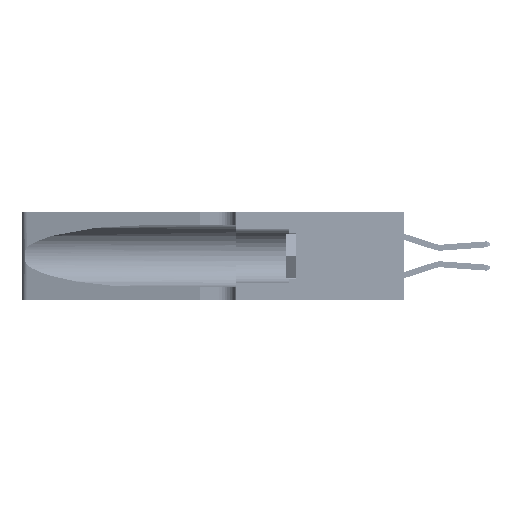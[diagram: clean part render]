
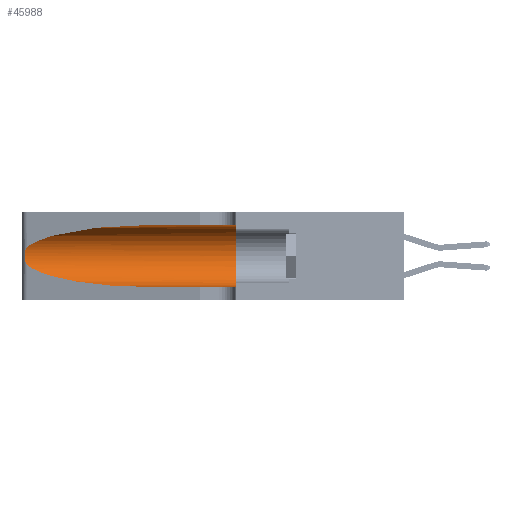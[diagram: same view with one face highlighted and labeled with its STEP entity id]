
A CAD part, left-side view. The second image highlights one B-rep face of the part: STEP entity #45988.
In plain terms, the highlighted cylindrical face has radius 3.308 mm (diameter 6.617 mm), a partial arc.
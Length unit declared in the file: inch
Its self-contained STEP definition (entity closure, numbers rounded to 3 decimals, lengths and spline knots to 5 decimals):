
#150 = CARTESIAN_POINT ( 'NONE',  ( 0.1305, 0.72297, 0.05475 ) ) ;
#905 = CARTESIAN_POINT ( 'NONE',  ( 0.25487, 1.22718, 0.14631 ) ) ;
#2768 = DIRECTION ( 'NONE',  ( 0., 0., 1. ) ) ;
#3040 = DIRECTION ( 'NONE',  ( 0., -1., 0. ) ) ;
#4184 = ORIENTED_EDGE ( 'NONE', *, *, #7627, .T. ) ;
#4466 = FACE_OUTER_BOUND ( 'NONE', #8411, .T. ) ;
#5339 = EDGE_CURVE ( 'NONE', #33217, #45054, #44253, .T. ) ;
#6113 = CARTESIAN_POINT ( 'NONE',  ( 0.25555, 1.22993, 0.14849 ) ) ;
#6825 = DIRECTION ( 'NONE',  ( 0., 0., -1. ) ) ;
#7461 = ORIENTED_EDGE ( 'NONE', *, *, #21922, .F. ) ;
#7483 = EDGE_CURVE ( 'NONE', #41468, #37640, #28538, .T. ) ;
#7627 = EDGE_CURVE ( 'NONE', #37640, #44772, #17730, .T. ) ;
#8411 = EDGE_LOOP ( 'NONE', ( #37162, #33918, #4184, #10391, #7461, #30241 ) ) ;
#8842 = DIRECTION ( 'NONE',  ( 0., -1., 0. ) ) ;
#9615 = VERTEX_POINT ( 'NONE', #32115 ) ;
#10391 = ORIENTED_EDGE ( 'NONE', *, *, #46859, .T. ) ;
#10669 = CARTESIAN_POINT ( 'NONE',  ( 0.25639, 1.23186, 0.15144 ) ) ;
#10843 = VECTOR ( 'NONE', #31134, 39.37008 ) ;
#11006 = CARTESIAN_POINT ( 'NONE',  ( 0.25555, 1.22994, 0.2215 ) ) ;
#11738 = CARTESIAN_POINT ( 'NONE',  ( 0.1305, 0.72297, 0.31525 ) ) ;
#15997 = CARTESIAN_POINT ( 'NONE',  ( 0.18966, 0.96281, 0.31525 ) ) ;
#16073 = EDGE_CURVE ( 'NONE', #33217, #41468, #32940, .T. ) ;
#16273 = VECTOR ( 'NONE', #8842, 39.37008 ) ;
#16305 = CARTESIAN_POINT ( 'NONE',  ( 0.1305, 1.61858, 0.05475 ) ) ;
#17011 = CARTESIAN_POINT ( 'NONE',  ( 0.1305, 0.72297, 0.31525 ) ) ;
#17193 = CARTESIAN_POINT ( 'NONE',  ( 0.25487, 1.22718, 0.22369 ) ) ;
#17338 = CIRCLE ( 'NONE', #37780, 0.13025 ) ;
#17730 =( BOUNDED_CURVE ( )  B_SPLINE_CURVE ( 3, ( #905, #27064, #31245, #42134 ),
 .UNSPECIFIED., .F., .F. ) 
 B_SPLINE_CURVE_WITH_KNOTS ( ( 4, 4 ),
 ( 3.44316, 4.71239 ),
 .UNSPECIFIED. ) 
 CURVE ( )  GEOMETRIC_REPRESENTATION_ITEM ( )  RATIONAL_B_SPLINE_CURVE ( ( 1., 0.87, 0.87, 1. ) ) 
 REPRESENTATION_ITEM ( '' )  );
#17924 = CARTESIAN_POINT ( 'NONE',  ( 0.1305, 1.61858, 0.185 ) ) ;
#18220 = CARTESIAN_POINT ( 'NONE',  ( 0.25789, 1.23486, 0.15765 ) ) ;
#18898 = CARTESIAN_POINT ( 'NONE',  ( 0.26017, 1.23833, 0.17102 ) ) ;
#21922 = EDGE_CURVE ( 'NONE', #45054, #9615, #17338, .T. ) ;
#22073 = CARTESIAN_POINT ( 'NONE',  ( 0.25487, 1.22718, 0.22369 ) ) ;
#22604 = CYLINDRICAL_SURFACE ( 'NONE', #29586, 0.13025 ) ;
#23156 = CARTESIAN_POINT ( 'NONE',  ( 0.25487, 1.22718, 0.22369 ) ) ;
#24676 = CARTESIAN_POINT ( 'NONE',  ( 0.1305, 0.35, 0.31525 ) ) ;
#27064 = CARTESIAN_POINT ( 'NONE',  ( 0.2373, 1.15595, 0.08982 ) ) ;
#28134 = CARTESIAN_POINT ( 'NONE',  ( 0.26075, 1.23896, 0.19203 ) ) ;
#28538 = B_SPLINE_CURVE_WITH_KNOTS ( 'NONE', 3,
 ( #22073, #11006, #30085, #45198, #34129, #37525, #28134, #32315, #18898, #39122, #18220, #10669, #6113, #37573 ),
 .UNSPECIFIED., .F., .F.,
 ( 4, 2, 2, 2, 2, 2, 4 ),
 ( 0., 0.00027, 0.00053, 0.00107, 0.0016, 0.00187, 0.00214 ),
 .UNSPECIFIED. ) ;
#28774 = DIRECTION ( 'NONE',  ( 0., 1., 0. ) ) ;
#29586 = AXIS2_PLACEMENT_3D ( 'NONE', #17924, #3040, #6825 ) ;
#30085 = CARTESIAN_POINT ( 'NONE',  ( 0.25639, 1.23184, 0.21858 ) ) ;
#30241 = ORIENTED_EDGE ( 'NONE', *, *, #5339, .F. ) ;
#30836 = CARTESIAN_POINT ( 'NONE',  ( 0.2373, 1.15595, 0.28018 ) ) ;
#31134 = DIRECTION ( 'NONE',  ( 0., -1., 0. ) ) ;
#31245 = CARTESIAN_POINT ( 'NONE',  ( 0.18966, 0.96281, 0.05475 ) ) ;
#32115 = CARTESIAN_POINT ( 'NONE',  ( 0.1305, 0.35, 0.05475 ) ) ;
#32315 = CARTESIAN_POINT ( 'NONE',  ( 0.26075, 1.23896, 0.178 ) ) ;
#32940 =( BOUNDED_CURVE ( )  B_SPLINE_CURVE ( 3, ( #11738, #15997, #30836, #23156 ),
 .UNSPECIFIED., .F., .F. ) 
 B_SPLINE_CURVE_WITH_KNOTS ( ( 4, 4 ),
 ( 1.5708, 2.84003 ),
 .UNSPECIFIED. ) 
 CURVE ( )  GEOMETRIC_REPRESENTATION_ITEM ( )  RATIONAL_B_SPLINE_CURVE ( ( 1., 0.87, 0.87, 1. ) ) 
 REPRESENTATION_ITEM ( '' )  );
#33217 = VERTEX_POINT ( 'NONE', #17011 ) ;
#33918 = ORIENTED_EDGE ( 'NONE', *, *, #7483, .T. ) ;
#34129 = CARTESIAN_POINT ( 'NONE',  ( 0.25854, 1.2359, 0.20912 ) ) ;
#37162 = ORIENTED_EDGE ( 'NONE', *, *, #16073, .T. ) ;
#37525 = CARTESIAN_POINT ( 'NONE',  ( 0.26018, 1.23835, 0.19895 ) ) ;
#37573 = CARTESIAN_POINT ( 'NONE',  ( 0.25487, 1.22718, 0.14631 ) ) ;
#37640 = VERTEX_POINT ( 'NONE', #37831 ) ;
#37780 = AXIS2_PLACEMENT_3D ( 'NONE', #43861, #28774, #2768 ) ;
#37831 = CARTESIAN_POINT ( 'NONE',  ( 0.25487, 1.22718, 0.14631 ) ) ;
#39122 = CARTESIAN_POINT ( 'NONE',  ( 0.25856, 1.23593, 0.16098 ) ) ;
#40778 = CARTESIAN_POINT ( 'NONE',  ( 0.1305, 1.61858, 0.31525 ) ) ;
#41468 = VERTEX_POINT ( 'NONE', #17193 ) ;
#42134 = CARTESIAN_POINT ( 'NONE',  ( 0.1305, 0.72297, 0.05475 ) ) ;
#43861 = CARTESIAN_POINT ( 'NONE',  ( 0.1305, 0.35, 0.185 ) ) ;
#44088 = LINE ( 'NONE', #16305, #10843 ) ;
#44253 = LINE ( 'NONE', #40778, #16273 ) ;
#44772 = VERTEX_POINT ( 'NONE', #150 ) ;
#45054 = VERTEX_POINT ( 'NONE', #24676 ) ;
#45198 = CARTESIAN_POINT ( 'NONE',  ( 0.25787, 1.23484, 0.2124 ) ) ;
#45988 = ADVANCED_FACE ( 'NONE', ( #4466 ), #22604, .F. ) ;
#46859 = EDGE_CURVE ( 'NONE', #44772, #9615, #44088, .T. ) ;
